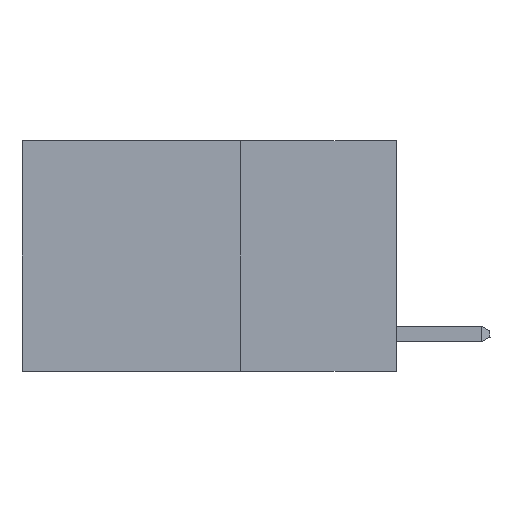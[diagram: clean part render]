
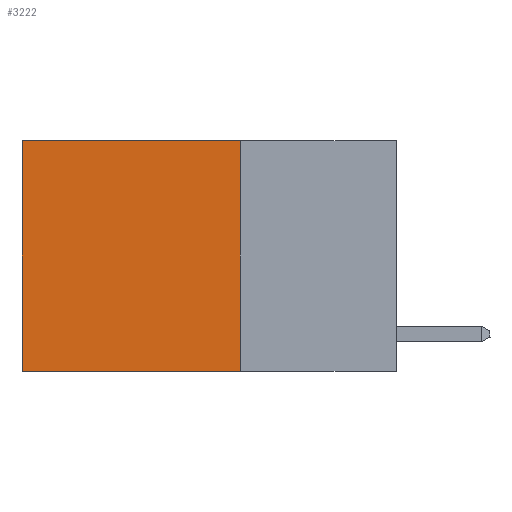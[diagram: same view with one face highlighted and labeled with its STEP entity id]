
A CAD part, left-side view. The second image highlights one B-rep face of the part: STEP entity #3222.
In plain terms, the highlighted planar face has unit normal (-1, 0, 0).
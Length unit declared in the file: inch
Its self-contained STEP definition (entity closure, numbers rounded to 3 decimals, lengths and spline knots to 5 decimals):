
#245 = DIRECTION ( 'NONE',  ( 0., 1., 0. ) ) ;
#251 = VERTEX_POINT ( 'NONE', #872 ) ;
#872 = CARTESIAN_POINT ( 'NONE',  ( 0.2625, 0.6, -0.37 ) ) ;
#1023 = CARTESIAN_POINT ( 'NONE',  ( 0.2625, 0.25, 0. ) ) ;
#1193 = DIRECTION ( 'NONE',  ( 0., 1., 0. ) ) ;
#1451 = EDGE_LOOP ( 'NONE', ( #4224, #1748, #2655, #2964 ) ) ;
#1748 = ORIENTED_EDGE ( 'NONE', *, *, #7481, .F. ) ;
#1784 = PLANE ( 'NONE',  #6085 ) ;
#1841 = VERTEX_POINT ( 'NONE', #2411 ) ;
#1939 = DIRECTION ( 'NONE',  ( 0., 0., -1. ) ) ;
#2063 = DIRECTION ( 'NONE',  ( 0., 0., -1. ) ) ;
#2262 = CARTESIAN_POINT ( 'NONE',  ( 0.2625, 0.25, -0.37 ) ) ;
#2339 = VECTOR ( 'NONE', #2063, 39.37008 ) ;
#2384 = LINE ( 'NONE', #7343, #5023 ) ;
#2411 = CARTESIAN_POINT ( 'NONE',  ( 0.2625, 0.6, 0. ) ) ;
#2580 = VERTEX_POINT ( 'NONE', #2262 ) ;
#2655 = ORIENTED_EDGE ( 'NONE', *, *, #5193, .F. ) ;
#2964 = ORIENTED_EDGE ( 'NONE', *, *, #3147, .T. ) ;
#3147 = EDGE_CURVE ( 'NONE', #5055, #1841, #7259, .T. ) ;
#3222 = ADVANCED_FACE ( 'NONE', ( #8058 ), #1784, .F. ) ;
#3292 = LINE ( 'NONE', #5555, #2339 ) ;
#3440 = VECTOR ( 'NONE', #245, 39.37008 ) ;
#3691 = DIRECTION ( 'NONE',  ( 1., 0., 0. ) ) ;
#4224 = ORIENTED_EDGE ( 'NONE', *, *, #6432, .T. ) ;
#4568 = CARTESIAN_POINT ( 'NONE',  ( 0.2625, 0.25, 0. ) ) ;
#5023 = VECTOR ( 'NONE', #1193, 39.37008 ) ;
#5055 = VERTEX_POINT ( 'NONE', #8675 ) ;
#5193 = EDGE_CURVE ( 'NONE', #5055, #2580, #5432, .T. ) ;
#5334 = CARTESIAN_POINT ( 'NONE',  ( 0.2625, 0.25, 0. ) ) ;
#5432 = LINE ( 'NONE', #5334, #5523 ) ;
#5523 = VECTOR ( 'NONE', #1939, 39.37008 ) ;
#5555 = CARTESIAN_POINT ( 'NONE',  ( 0.2625, 0.6, 0. ) ) ;
#6085 = AXIS2_PLACEMENT_3D ( 'NONE', #4568, #3691, #6549 ) ;
#6432 = EDGE_CURVE ( 'NONE', #1841, #251, #3292, .T. ) ;
#6549 = DIRECTION ( 'NONE',  ( 0., 0., -1. ) ) ;
#7259 = LINE ( 'NONE', #1023, #3440 ) ;
#7343 = CARTESIAN_POINT ( 'NONE',  ( 0.2625, 0.25, -0.37 ) ) ;
#7481 = EDGE_CURVE ( 'NONE', #2580, #251, #2384, .T. ) ;
#8058 = FACE_OUTER_BOUND ( 'NONE', #1451, .T. ) ;
#8675 = CARTESIAN_POINT ( 'NONE',  ( 0.2625, 0.25, 0. ) ) ;
